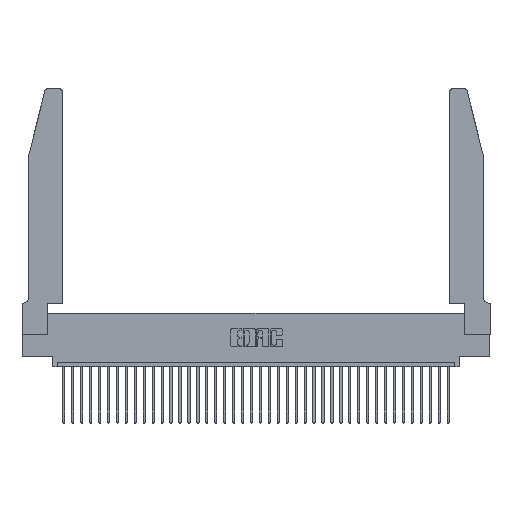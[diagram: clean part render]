
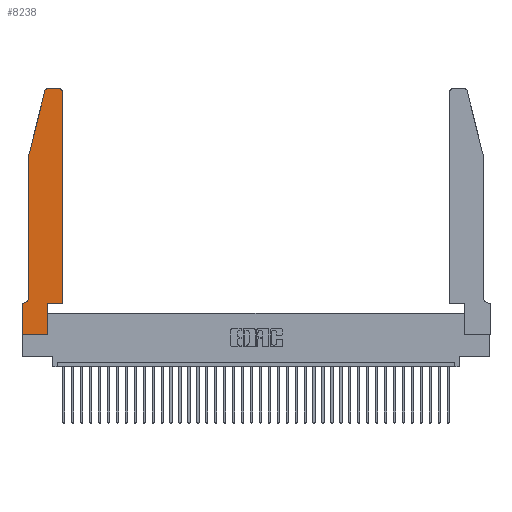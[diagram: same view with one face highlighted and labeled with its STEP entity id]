
A CAD part, top view. The second image highlights one B-rep face of the part: STEP entity #8238.
In plain terms, the highlighted planar face has unit normal (0, 0, 1).
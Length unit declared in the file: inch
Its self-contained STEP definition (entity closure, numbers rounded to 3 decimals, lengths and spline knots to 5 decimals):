
#352 = DIRECTION ( 'NONE',  ( -0.239, -0.971, 0. ) ) ;
#747 = CIRCLE ( 'NONE', #22124, 0.07 ) ;
#851 = LINE ( 'NONE', #19827, #34614 ) ;
#1227 = CARTESIAN_POINT ( 'NONE',  ( 0.4205, 2.75, 0.37 ) ) ;
#1477 = CARTESIAN_POINT ( 'NONE',  ( 0.2865, 0.35, 0.37 ) ) ;
#1658 = EDGE_CURVE ( 'NONE', #21243, #15581, #11159, .T. ) ;
#1708 = CARTESIAN_POINT ( 'NONE',  ( 0.4505, 0.35, 0.37 ) ) ;
#2025 = DIRECTION ( 'NONE',  ( 0., 0., -1. ) ) ;
#2137 = VERTEX_POINT ( 'NONE', #7640 ) ;
#3597 = AXIS2_PLACEMENT_3D ( 'NONE', #27998, #23735, #26641 ) ;
#3659 = CARTESIAN_POINT ( 'NONE',  ( 0.0055, 0.35, 0.37 ) ) ;
#4165 = AXIS2_PLACEMENT_3D ( 'NONE', #33768, #36706, #10596 ) ;
#4774 = CARTESIAN_POINT ( 'NONE',  ( 0.0755, 0.42, 0.37 ) ) ;
#5058 = LINE ( 'NONE', #16145, #27396 ) ;
#5236 = DIRECTION ( 'NONE',  ( -1., 0., 0. ) ) ;
#5378 = CARTESIAN_POINT ( 'NONE',  ( 0.4505, 0.35, 0.37 ) ) ;
#5457 = CARTESIAN_POINT ( 'NONE',  ( 0., 0.35, 0.37 ) ) ;
#6570 = EDGE_CURVE ( 'NONE', #31864, #32029, #13360, .T. ) ;
#6682 = DIRECTION ( 'NONE',  ( 0., -1., 0. ) ) ;
#7260 = ORIENTED_EDGE ( 'NONE', *, *, #31342, .T. ) ;
#7341 = ORIENTED_EDGE ( 'NONE', *, *, #29723, .T. ) ;
#7358 = VECTOR ( 'NONE', #27763, 39.37008 ) ;
#7640 = CARTESIAN_POINT ( 'NONE',  ( 0.0755, 2., 0.37 ) ) ;
#7654 = CARTESIAN_POINT ( 'NONE',  ( 0.0055, 0.42, 0.37 ) ) ;
#7656 = ORIENTED_EDGE ( 'NONE', *, *, #26392, .T. ) ;
#7856 = LINE ( 'NONE', #10540, #7358 ) ;
#8238 = ADVANCED_FACE ( 'NONE', ( #16441 ), #25036, .T. ) ;
#9094 = CARTESIAN_POINT ( 'NONE',  ( 0.2865, 0.35, 0.37 ) ) ;
#9097 = VECTOR ( 'NONE', #9525, 39.37008 ) ;
#9215 = VECTOR ( 'NONE', #15012, 39.37008 ) ;
#9242 = VECTOR ( 'NONE', #14303, 39.37008 ) ;
#9525 = DIRECTION ( 'NONE',  ( -1., 0., 0. ) ) ;
#9554 = ORIENTED_EDGE ( 'NONE', *, *, #6570, .T. ) ;
#10010 = CARTESIAN_POINT ( 'NONE',  ( 0.284, 2.72, 0.37 ) ) ;
#10540 = CARTESIAN_POINT ( 'NONE',  ( 0.2605, 2.75, 0.37 ) ) ;
#10568 = LINE ( 'NONE', #12390, #26073 ) ;
#10596 = DIRECTION ( 'NONE',  ( 1., 0., 0. ) ) ;
#10674 = EDGE_CURVE ( 'NONE', #33840, #28211, #29511, .T. ) ;
#10911 = DIRECTION ( 'NONE',  ( 0., -1., 0. ) ) ;
#10990 = LINE ( 'NONE', #12598, #9097 ) ;
#11144 = EDGE_CURVE ( 'NONE', #15581, #14715, #851, .T. ) ;
#11159 = LINE ( 'NONE', #16256, #26626 ) ;
#11222 = CARTESIAN_POINT ( 'NONE',  ( 0.2865, 0., 0.37 ) ) ;
#12390 = CARTESIAN_POINT ( 'NONE',  ( 0.0755, 2., 0.37 ) ) ;
#12502 = ORIENTED_EDGE ( 'NONE', *, *, #1658, .T. ) ;
#12598 = CARTESIAN_POINT ( 'NONE',  ( 0.0755, 0.35, 0.37 ) ) ;
#13360 = LINE ( 'NONE', #23730, #9215 ) ;
#14303 = DIRECTION ( 'NONE',  ( 0., 1., 0. ) ) ;
#14715 = VERTEX_POINT ( 'NONE', #11222 ) ;
#15012 = DIRECTION ( 'NONE',  ( 1., 0., 0. ) ) ;
#15581 = VERTEX_POINT ( 'NONE', #29941 ) ;
#16145 = CARTESIAN_POINT ( 'NONE',  ( 0.0755, 2., 0.37 ) ) ;
#16256 = CARTESIAN_POINT ( 'NONE',  ( 0., 0., 0.37 ) ) ;
#16270 = ORIENTED_EDGE ( 'NONE', *, *, #17920, .T. ) ;
#16322 = ORIENTED_EDGE ( 'NONE', *, *, #37646, .T. ) ;
#16441 = FACE_OUTER_BOUND ( 'NONE', #21092, .T. ) ;
#17327 = VECTOR ( 'NONE', #36527, 39.37008 ) ;
#17394 = CARTESIAN_POINT ( 'NONE',  ( 0.25487, 2.72718, 0.37 ) ) ;
#17920 = EDGE_CURVE ( 'NONE', #28211, #21265, #7856, .T. ) ;
#18598 = DIRECTION ( 'NONE',  ( 1., 0., 0. ) ) ;
#19827 = CARTESIAN_POINT ( 'NONE',  ( 0., 0., 0.37 ) ) ;
#19842 = VERTEX_POINT ( 'NONE', #4774 ) ;
#21092 = EDGE_LOOP ( 'NONE', ( #16270, #23777, #7656, #22333, #16322, #7260, #12502, #30851, #32235, #9554, #7341, #37232 ) ) ;
#21243 = VERTEX_POINT ( 'NONE', #5457 ) ;
#21265 = VERTEX_POINT ( 'NONE', #31470 ) ;
#21625 = CARTESIAN_POINT ( 'NONE',  ( 0.4505, 2.72, 0.37 ) ) ;
#21659 = DIRECTION ( 'NONE',  ( 0., 0., 1. ) ) ;
#22124 = AXIS2_PLACEMENT_3D ( 'NONE', #7654, #2025, #5236 ) ;
#22333 = ORIENTED_EDGE ( 'NONE', *, *, #31980, .T. ) ;
#23730 = CARTESIAN_POINT ( 'NONE',  ( 0.4505, 0.35, 0.37 ) ) ;
#23735 = DIRECTION ( 'NONE',  ( 0., 0., 1. ) ) ;
#23777 = ORIENTED_EDGE ( 'NONE', *, *, #25264, .T. ) ;
#23899 = LINE ( 'NONE', #5378, #9242 ) ;
#25036 = PLANE ( 'NONE',  #3597 ) ;
#25264 = EDGE_CURVE ( 'NONE', #21265, #27225, #30033, .T. ) ;
#26073 = VECTOR ( 'NONE', #352, 39.37008 ) ;
#26392 = EDGE_CURVE ( 'NONE', #27225, #2137, #10568, .T. ) ;
#26626 = VECTOR ( 'NONE', #10911, 39.37008 ) ;
#26641 = DIRECTION ( 'NONE',  ( 1., 0., 0. ) ) ;
#27225 = VERTEX_POINT ( 'NONE', #17394 ) ;
#27396 = VECTOR ( 'NONE', #6682, 39.37008 ) ;
#27763 = DIRECTION ( 'NONE',  ( -1., 0., 0. ) ) ;
#27998 = CARTESIAN_POINT ( 'NONE',  ( 0., 0.35, 0.37 ) ) ;
#28211 = VERTEX_POINT ( 'NONE', #1227 ) ;
#29175 = LINE ( 'NONE', #1477, #17327 ) ;
#29511 = CIRCLE ( 'NONE', #4165, 0.03 ) ;
#29723 = EDGE_CURVE ( 'NONE', #32029, #33840, #23899, .T. ) ;
#29941 = CARTESIAN_POINT ( 'NONE',  ( 0., 0., 0.37 ) ) ;
#30033 = CIRCLE ( 'NONE', #32754, 0.03 ) ;
#30851 = ORIENTED_EDGE ( 'NONE', *, *, #11144, .T. ) ;
#31342 = EDGE_CURVE ( 'NONE', #37463, #21243, #10990, .T. ) ;
#31470 = CARTESIAN_POINT ( 'NONE',  ( 0.284, 2.75, 0.37 ) ) ;
#31864 = VERTEX_POINT ( 'NONE', #9094 ) ;
#31980 = EDGE_CURVE ( 'NONE', #2137, #19842, #5058, .T. ) ;
#32029 = VERTEX_POINT ( 'NONE', #1708 ) ;
#32235 = ORIENTED_EDGE ( 'NONE', *, *, #36359, .T. ) ;
#32754 = AXIS2_PLACEMENT_3D ( 'NONE', #10010, #21659, #35985 ) ;
#33768 = CARTESIAN_POINT ( 'NONE',  ( 0.4205, 2.72, 0.37 ) ) ;
#33840 = VERTEX_POINT ( 'NONE', #21625 ) ;
#34614 = VECTOR ( 'NONE', #18598, 39.37008 ) ;
#35985 = DIRECTION ( 'NONE',  ( 1., 0., 0. ) ) ;
#36359 = EDGE_CURVE ( 'NONE', #14715, #31864, #29175, .T. ) ;
#36527 = DIRECTION ( 'NONE',  ( 0., 1., 0. ) ) ;
#36706 = DIRECTION ( 'NONE',  ( 0., 0., 1. ) ) ;
#37232 = ORIENTED_EDGE ( 'NONE', *, *, #10674, .T. ) ;
#37463 = VERTEX_POINT ( 'NONE', #3659 ) ;
#37646 = EDGE_CURVE ( 'NONE', #19842, #37463, #747, .T. ) ;
